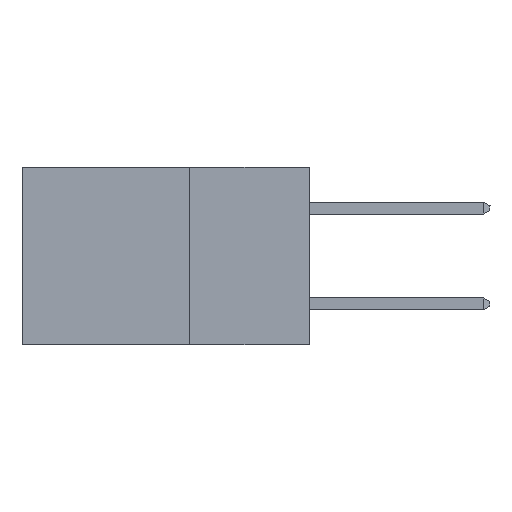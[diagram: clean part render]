
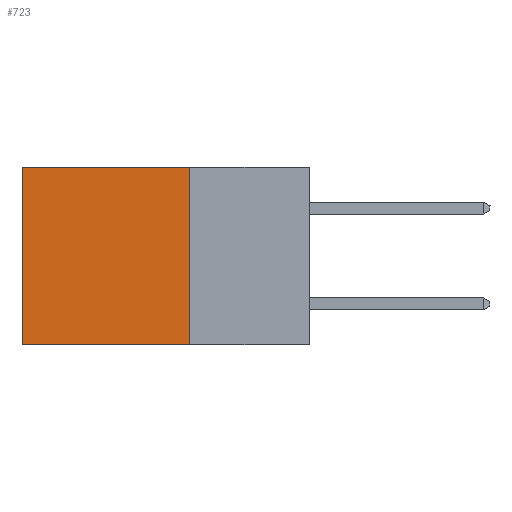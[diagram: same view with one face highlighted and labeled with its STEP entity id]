
A CAD part, left-side view. The second image highlights one B-rep face of the part: STEP entity #723.
In plain terms, the highlighted planar face has unit normal (-1, 0, 0).
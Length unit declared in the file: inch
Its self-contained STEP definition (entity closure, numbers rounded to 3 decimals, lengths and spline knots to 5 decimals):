
#223 = CARTESIAN_POINT ( 'NONE',  ( 0.2875, 0.25, 0. ) ) ;
#366 = CARTESIAN_POINT ( 'NONE',  ( 0.2875, 0.6, 0. ) ) ;
#668 = DIRECTION ( 'NONE',  ( 0., 0., -1. ) ) ;
#723 = ADVANCED_FACE ( 'NONE', ( #11676 ), #11603, .F. ) ;
#1277 = VERTEX_POINT ( 'NONE', #366 ) ;
#1437 = VERTEX_POINT ( 'NONE', #10911 ) ;
#2487 = EDGE_CURVE ( 'NONE', #9122, #1277, #12327, .T. ) ;
#2572 = DIRECTION ( 'NONE',  ( 1., 0., 0. ) ) ;
#3209 = VECTOR ( 'NONE', #5993, 39.37008 ) ;
#3210 = CARTESIAN_POINT ( 'NONE',  ( 0.2875, 0.25, -0.37 ) ) ;
#3896 = ORIENTED_EDGE ( 'NONE', *, *, #11986, .F. ) ;
#4128 = CARTESIAN_POINT ( 'NONE',  ( 0.2875, 0.25, -0.37 ) ) ;
#4695 = LINE ( 'NONE', #5874, #16364 ) ;
#5874 = CARTESIAN_POINT ( 'NONE',  ( 0.2875, 0.25, 0. ) ) ;
#5993 = DIRECTION ( 'NONE',  ( 0., 1., 0. ) ) ;
#7032 = CARTESIAN_POINT ( 'NONE',  ( 0.2875, 0.6, 0. ) ) ;
#7090 = EDGE_CURVE ( 'NONE', #1277, #1437, #10867, .T. ) ;
#7250 = VECTOR ( 'NONE', #8021, 39.37008 ) ;
#7462 = VECTOR ( 'NONE', #14396, 39.37008 ) ;
#8021 = DIRECTION ( 'NONE',  ( 0., 0., -1. ) ) ;
#8802 = ORIENTED_EDGE ( 'NONE', *, *, #11484, .F. ) ;
#9122 = VERTEX_POINT ( 'NONE', #16099 ) ;
#9990 = VERTEX_POINT ( 'NONE', #3210 ) ;
#10294 = ORIENTED_EDGE ( 'NONE', *, *, #2487, .T. ) ;
#10479 = LINE ( 'NONE', #4128, #7462 ) ;
#10867 = LINE ( 'NONE', #7032, #7250 ) ;
#10911 = CARTESIAN_POINT ( 'NONE',  ( 0.2875, 0.6, -0.37 ) ) ;
#11356 = DIRECTION ( 'NONE',  ( 0., 0., -1. ) ) ;
#11484 = EDGE_CURVE ( 'NONE', #9990, #1437, #10479, .T. ) ;
#11603 = PLANE ( 'NONE',  #16092 ) ;
#11676 = FACE_OUTER_BOUND ( 'NONE', #13452, .T. ) ;
#11986 = EDGE_CURVE ( 'NONE', #9122, #9990, #4695, .T. ) ;
#12327 = LINE ( 'NONE', #13657, #3209 ) ;
#12943 = ORIENTED_EDGE ( 'NONE', *, *, #7090, .T. ) ;
#13452 = EDGE_LOOP ( 'NONE', ( #12943, #8802, #3896, #10294 ) ) ;
#13657 = CARTESIAN_POINT ( 'NONE',  ( 0.2875, 0.25, 0. ) ) ;
#14396 = DIRECTION ( 'NONE',  ( 0., 1., 0. ) ) ;
#16092 = AXIS2_PLACEMENT_3D ( 'NONE', #223, #2572, #11356 ) ;
#16099 = CARTESIAN_POINT ( 'NONE',  ( 0.2875, 0.25, 0. ) ) ;
#16364 = VECTOR ( 'NONE', #668, 39.37008 ) ;
